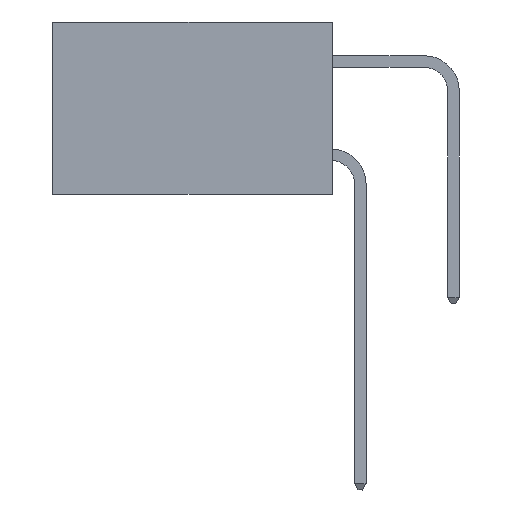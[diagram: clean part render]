
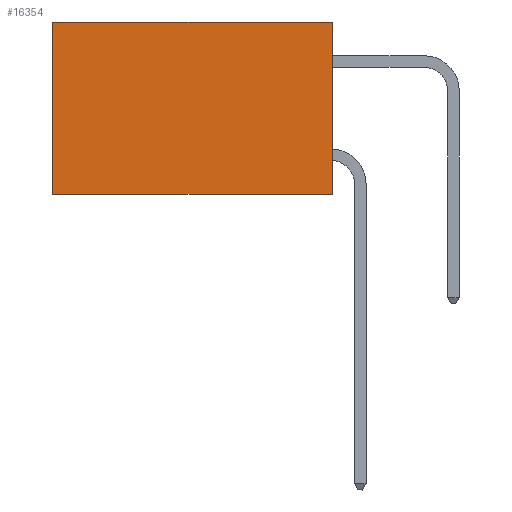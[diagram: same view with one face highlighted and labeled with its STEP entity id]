
A CAD part, left-side view. The second image highlights one B-rep face of the part: STEP entity #16354.
In plain terms, the highlighted planar face has unit normal (-1, 0, 0).
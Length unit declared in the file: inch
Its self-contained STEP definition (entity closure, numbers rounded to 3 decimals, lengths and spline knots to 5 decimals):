
#496 = ORIENTED_EDGE ( 'NONE', *, *, #26687, .F. ) ;
#2260 = DIRECTION ( 'NONE',  ( 0., 0., -1. ) ) ;
#2327 = VERTEX_POINT ( 'NONE', #10749 ) ;
#2783 = VECTOR ( 'NONE', #16709, 39.37008 ) ;
#4829 = EDGE_CURVE ( 'NONE', #13664, #2327, #29792, .T. ) ;
#5344 = FACE_OUTER_BOUND ( 'NONE', #30282, .T. ) ;
#5929 = EDGE_CURVE ( 'NONE', #18996, #8517, #19042, .T. ) ;
#6029 = CARTESIAN_POINT ( 'NONE',  ( 0.298, 0., -0.37 ) ) ;
#6530 = EDGE_CURVE ( 'NONE', #2327, #8517, #29705, .T. ) ;
#8003 = CARTESIAN_POINT ( 'NONE',  ( 0.298, 0., 0. ) ) ;
#8517 = VERTEX_POINT ( 'NONE', #12550 ) ;
#10741 = CARTESIAN_POINT ( 'NONE',  ( 0.298, 0., 0. ) ) ;
#10749 = CARTESIAN_POINT ( 'NONE',  ( 0.298, 0.6, 0. ) ) ;
#12550 = CARTESIAN_POINT ( 'NONE',  ( 0.298, 0.6, -0.37 ) ) ;
#13664 = VERTEX_POINT ( 'NONE', #19064 ) ;
#15270 = LINE ( 'NONE', #8003, #19186 ) ;
#16354 = ADVANCED_FACE ( 'NONE', ( #5344 ), #27730, .F. ) ;
#16709 = DIRECTION ( 'NONE',  ( 0., 0., -1. ) ) ;
#17085 = AXIS2_PLACEMENT_3D ( 'NONE', #32790, #17390, #2260 ) ;
#17390 = DIRECTION ( 'NONE',  ( 1., 0., 0. ) ) ;
#18996 = VERTEX_POINT ( 'NONE', #31839 ) ;
#19042 = LINE ( 'NONE', #6029, #27792 ) ;
#19064 = CARTESIAN_POINT ( 'NONE',  ( 0.298, 0., 0. ) ) ;
#19186 = VECTOR ( 'NONE', #23544, 39.37008 ) ;
#19707 = ORIENTED_EDGE ( 'NONE', *, *, #6530, .T. ) ;
#23423 = DIRECTION ( 'NONE',  ( 0., 1., 0. ) ) ;
#23544 = DIRECTION ( 'NONE',  ( 0., 0., -1. ) ) ;
#26520 = DIRECTION ( 'NONE',  ( 0., 1., 0. ) ) ;
#26648 = VECTOR ( 'NONE', #23423, 39.37008 ) ;
#26687 = EDGE_CURVE ( 'NONE', #13664, #18996, #15270, .T. ) ;
#27074 = ORIENTED_EDGE ( 'NONE', *, *, #5929, .F. ) ;
#27730 = PLANE ( 'NONE',  #17085 ) ;
#27792 = VECTOR ( 'NONE', #26520, 39.37008 ) ;
#29705 = LINE ( 'NONE', #32025, #2783 ) ;
#29792 = LINE ( 'NONE', #10741, #26648 ) ;
#29879 = ORIENTED_EDGE ( 'NONE', *, *, #4829, .T. ) ;
#30282 = EDGE_LOOP ( 'NONE', ( #19707, #27074, #496, #29879 ) ) ;
#31839 = CARTESIAN_POINT ( 'NONE',  ( 0.298, 0., -0.37 ) ) ;
#32025 = CARTESIAN_POINT ( 'NONE',  ( 0.298, 0.6, 0. ) ) ;
#32790 = CARTESIAN_POINT ( 'NONE',  ( 0.298, 0., 0. ) ) ;
